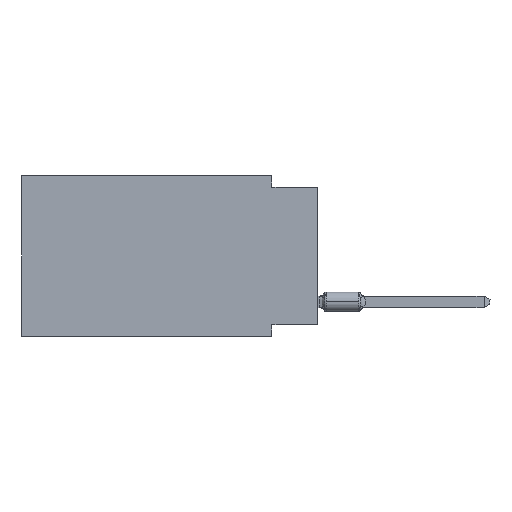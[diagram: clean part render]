
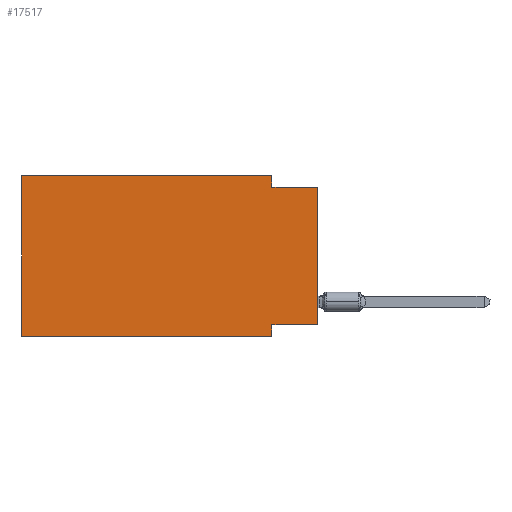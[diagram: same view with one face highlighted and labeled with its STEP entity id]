
A CAD part, left-side view. The second image highlights one B-rep face of the part: STEP entity #17517.
In plain terms, the highlighted planar face has unit normal (-1, 0, 0).
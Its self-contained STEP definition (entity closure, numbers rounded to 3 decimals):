
#144 = LINE ( 'NONE', #5102, #7402 ) ;
#312 = CARTESIAN_POINT ( 'NONE',  ( 0., 16.383, -8.89 ) ) ;
#809 = VERTEX_POINT ( 'NONE', #15582 ) ;
#1436 = ORIENTED_EDGE ( 'NONE', *, *, #1942, .T. ) ;
#1603 = EDGE_CURVE ( 'NONE', #1719, #8520, #4005, .T. ) ;
#1719 = VERTEX_POINT ( 'NONE', #5988 ) ;
#1942 = EDGE_CURVE ( 'NONE', #809, #16082, #8530, .T. ) ;
#2265 = DIRECTION ( 'NONE',  ( 0., 0., -1. ) ) ;
#2839 = CARTESIAN_POINT ( 'NONE',  ( 0., 2.54, 0. ) ) ;
#3478 = ORIENTED_EDGE ( 'NONE', *, *, #20865, .F. ) ;
#4005 = LINE ( 'NONE', #18692, #9881 ) ;
#4094 = VERTEX_POINT ( 'NONE', #14250 ) ;
#4567 = VERTEX_POINT ( 'NONE', #6180 ) ;
#4593 = EDGE_CURVE ( 'NONE', #809, #4567, #144, .T. ) ;
#5102 = CARTESIAN_POINT ( 'NONE',  ( 0., 0., -8.255 ) ) ;
#5745 = VERTEX_POINT ( 'NONE', #17711 ) ;
#5788 = DIRECTION ( 'NONE',  ( 0., -1., 0. ) ) ;
#5878 = VECTOR ( 'NONE', #13908, 1000. ) ;
#5988 = CARTESIAN_POINT ( 'NONE',  ( 0., 16.383, 0. ) ) ;
#6180 = CARTESIAN_POINT ( 'NONE',  ( 0., 2.54, -8.255 ) ) ;
#6336 = VERTEX_POINT ( 'NONE', #15153 ) ;
#6506 = DIRECTION ( 'NONE',  ( 0., 0., 1. ) ) ;
#6759 = DIRECTION ( 'NONE',  ( 0., -1., 0. ) ) ;
#6765 = EDGE_LOOP ( 'NONE', ( #1436, #3478, #12248, #7979, #17819, #19257, #7799, #9946 ) ) ;
#7402 = VECTOR ( 'NONE', #16536, 1000. ) ;
#7799 = ORIENTED_EDGE ( 'NONE', *, *, #13228, .F. ) ;
#7979 = ORIENTED_EDGE ( 'NONE', *, *, #1603, .F. ) ;
#8520 = VERTEX_POINT ( 'NONE', #20540 ) ;
#8530 = LINE ( 'NONE', #16664, #15572 ) ;
#8616 = DIRECTION ( 'NONE',  ( 1., 0., 0. ) ) ;
#9382 = LINE ( 'NONE', #12649, #19461 ) ;
#9881 = VECTOR ( 'NONE', #5788, 1000. ) ;
#9903 = LINE ( 'NONE', #16334, #16091 ) ;
#9946 = ORIENTED_EDGE ( 'NONE', *, *, #4593, .F. ) ;
#10197 = CARTESIAN_POINT ( 'NONE',  ( 0., 16.383, 0. ) ) ;
#10432 = LINE ( 'NONE', #18661, #5878 ) ;
#10980 = LINE ( 'NONE', #2839, #19788 ) ;
#11276 = DIRECTION ( 'NONE',  ( 0., 0., -1. ) ) ;
#11571 = EDGE_CURVE ( 'NONE', #8520, #6336, #10980, .T. ) ;
#11844 = LINE ( 'NONE', #312, #18759 ) ;
#12248 = ORIENTED_EDGE ( 'NONE', *, *, #11571, .F. ) ;
#12649 = CARTESIAN_POINT ( 'NONE',  ( 0., 2.54, -8.89 ) ) ;
#13175 = DIRECTION ( 'NONE',  ( 0., 0., 1. ) ) ;
#13228 = EDGE_CURVE ( 'NONE', #4567, #4094, #9382, .T. ) ;
#13395 = EDGE_CURVE ( 'NONE', #5745, #1719, #9903, .T. ) ;
#13477 = PLANE ( 'NONE',  #15827 ) ;
#13908 = DIRECTION ( 'NONE',  ( 0., -1., 0. ) ) ;
#14250 = CARTESIAN_POINT ( 'NONE',  ( 0., 2.54, -8.89 ) ) ;
#15153 = CARTESIAN_POINT ( 'NONE',  ( 0., 2.54, -0.635 ) ) ;
#15572 = VECTOR ( 'NONE', #13175, 1000. ) ;
#15582 = CARTESIAN_POINT ( 'NONE',  ( 0., 0., -8.255 ) ) ;
#15827 = AXIS2_PLACEMENT_3D ( 'NONE', #10197, #8616, #2265 ) ;
#16082 = VERTEX_POINT ( 'NONE', #17275 ) ;
#16091 = VECTOR ( 'NONE', #6506, 1000. ) ;
#16334 = CARTESIAN_POINT ( 'NONE',  ( 0., 16.383, 0. ) ) ;
#16536 = DIRECTION ( 'NONE',  ( 0., 1., 0. ) ) ;
#16664 = CARTESIAN_POINT ( 'NONE',  ( 0., 0., 0. ) ) ;
#16748 = FACE_OUTER_BOUND ( 'NONE', #6765, .T. ) ;
#17275 = CARTESIAN_POINT ( 'NONE',  ( 0., 0., -0.635 ) ) ;
#17517 = ADVANCED_FACE ( 'NONE', ( #16748 ), #13477, .F. ) ;
#17711 = CARTESIAN_POINT ( 'NONE',  ( 0., 16.383, -8.89 ) ) ;
#17819 = ORIENTED_EDGE ( 'NONE', *, *, #13395, .F. ) ;
#18661 = CARTESIAN_POINT ( 'NONE',  ( 0., 0., -0.635 ) ) ;
#18692 = CARTESIAN_POINT ( 'NONE',  ( 0., 16.383, 0. ) ) ;
#18759 = VECTOR ( 'NONE', #6759, 1000. ) ;
#19257 = ORIENTED_EDGE ( 'NONE', *, *, #20064, .T. ) ;
#19461 = VECTOR ( 'NONE', #11276, 1000. ) ;
#19493 = DIRECTION ( 'NONE',  ( 0., 0., -1. ) ) ;
#19788 = VECTOR ( 'NONE', #19493, 1000. ) ;
#20064 = EDGE_CURVE ( 'NONE', #5745, #4094, #11844, .T. ) ;
#20540 = CARTESIAN_POINT ( 'NONE',  ( 0., 2.54, 0. ) ) ;
#20865 = EDGE_CURVE ( 'NONE', #6336, #16082, #10432, .T. ) ;
